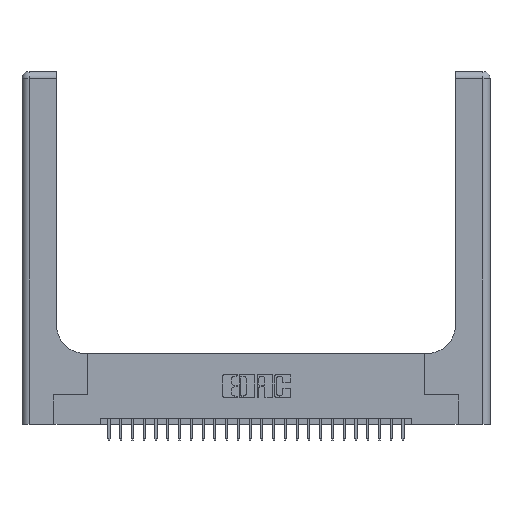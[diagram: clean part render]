
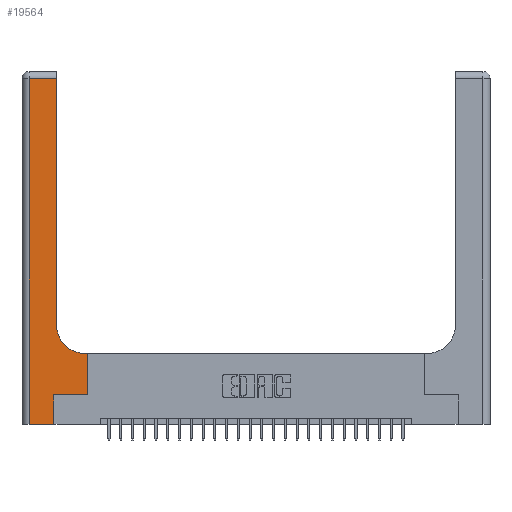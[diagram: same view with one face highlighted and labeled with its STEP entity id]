
A CAD part, top view. The second image highlights one B-rep face of the part: STEP entity #19564.
In plain terms, the highlighted planar face has unit normal (0, 0, 1).
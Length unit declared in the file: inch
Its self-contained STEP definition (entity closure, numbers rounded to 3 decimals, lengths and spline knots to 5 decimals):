
#420 = LINE ( 'NONE', #9033, #13982 ) ;
#2180 = LINE ( 'NONE', #6557, #15878 ) ;
#2312 = DIRECTION ( 'NONE',  ( -1., 0., 0. ) ) ;
#2355 = EDGE_CURVE ( 'NONE', #3383, #12355, #4065, .T. ) ;
#3005 = CARTESIAN_POINT ( 'NONE',  ( 0.5585, 0.6, 0.37 ) ) ;
#3383 = VERTEX_POINT ( 'NONE', #3005 ) ;
#4065 = LINE ( 'NONE', #10394, #23640 ) ;
#4343 = CARTESIAN_POINT ( 'NONE',  ( 0.269, 0., 0.37 ) ) ;
#4801 = CIRCLE ( 'NONE', #18750, 0.25 ) ;
#4947 = DIRECTION ( 'NONE',  ( 0., -1., 0. ) ) ;
#5912 = ORIENTED_EDGE ( 'NONE', *, *, #10742, .T. ) ;
#6061 = DIRECTION ( 'NONE',  ( 1., 0., 0. ) ) ;
#6250 = ORIENTED_EDGE ( 'NONE', *, *, #11276, .T. ) ;
#6557 = CARTESIAN_POINT ( 'NONE',  ( 0.269, 0., 0.37 ) ) ;
#6589 = CARTESIAN_POINT ( 'NONE',  ( 0.2915, 3., 0.37 ) ) ;
#6595 = EDGE_CURVE ( 'NONE', #12355, #13264, #4801, .T. ) ;
#6789 = LINE ( 'NONE', #21723, #9915 ) ;
#7069 = CARTESIAN_POINT ( 'NONE',  ( 0.5415, 0.85, 0.37 ) ) ;
#7431 = CARTESIAN_POINT ( 'NONE',  ( 0.5585, 0.25, 0.37 ) ) ;
#7703 = VECTOR ( 'NONE', #19252, 39.37008 ) ;
#8485 = CARTESIAN_POINT ( 'NONE',  ( 0.2915, 0.85, 0.37 ) ) ;
#8656 = DIRECTION ( 'NONE',  ( 0., 0., -1. ) ) ;
#9033 = CARTESIAN_POINT ( 'NONE',  ( 0., 0., 0.37 ) ) ;
#9044 = EDGE_CURVE ( 'NONE', #11188, #22941, #14479, .T. ) ;
#9915 = VECTOR ( 'NONE', #26227, 39.37008 ) ;
#10226 = DIRECTION ( 'NONE',  ( 1., 0., 0. ) ) ;
#10310 = ORIENTED_EDGE ( 'NONE', *, *, #14823, .T. ) ;
#10365 = CARTESIAN_POINT ( 'NONE',  ( 0., 3., 0.37 ) ) ;
#10394 = CARTESIAN_POINT ( 'NONE',  ( 0.2915, 0.6, 0.37 ) ) ;
#10742 = EDGE_CURVE ( 'NONE', #13264, #24520, #14878, .T. ) ;
#11186 = CARTESIAN_POINT ( 'NONE',  ( 0.2915, 2.94, 0.37 ) ) ;
#11188 = VERTEX_POINT ( 'NONE', #18520 ) ;
#11276 = EDGE_CURVE ( 'NONE', #20802, #11188, #2180, .T. ) ;
#11529 = EDGE_LOOP ( 'NONE', ( #5912, #10310, #25413, #22060, #6250, #22287, #21611, #18761, #16206 ) ) ;
#11717 = EDGE_CURVE ( 'NONE', #25289, #20802, #420, .T. ) ;
#12355 = VERTEX_POINT ( 'NONE', #26466 ) ;
#12738 = VECTOR ( 'NONE', #26748, 39.37008 ) ;
#13264 = VERTEX_POINT ( 'NONE', #8485 ) ;
#13982 = VECTOR ( 'NONE', #10226, 39.37008 ) ;
#14479 = LINE ( 'NONE', #20710, #26351 ) ;
#14733 = EDGE_CURVE ( 'NONE', #19718, #25289, #17744, .T. ) ;
#14823 = EDGE_CURVE ( 'NONE', #24520, #19718, #6789, .T. ) ;
#14878 = LINE ( 'NONE', #6589, #7703 ) ;
#15251 = DIRECTION ( 'NONE',  ( 0., 1., 0. ) ) ;
#15878 = VECTOR ( 'NONE', #15251, 39.37008 ) ;
#16206 = ORIENTED_EDGE ( 'NONE', *, *, #6595, .T. ) ;
#17053 = CARTESIAN_POINT ( 'NONE',  ( 0.06, 0., 0.37 ) ) ;
#17500 = VECTOR ( 'NONE', #4947, 39.37008 ) ;
#17744 = LINE ( 'NONE', #24397, #17500 ) ;
#18520 = CARTESIAN_POINT ( 'NONE',  ( 0.269, 0.25, 0.37 ) ) ;
#18619 = CARTESIAN_POINT ( 'NONE',  ( 0.06, 2.94, 0.37 ) ) ;
#18750 = AXIS2_PLACEMENT_3D ( 'NONE', #7069, #24282, #24694 ) ;
#18761 = ORIENTED_EDGE ( 'NONE', *, *, #2355, .T. ) ;
#18976 = DIRECTION ( 'NONE',  ( -1., 0., 0. ) ) ;
#19252 = DIRECTION ( 'NONE',  ( 0., 1., 0. ) ) ;
#19564 = ADVANCED_FACE ( 'NONE', ( #23201 ), #23476, .F. ) ;
#19718 = VERTEX_POINT ( 'NONE', #18619 ) ;
#20395 = LINE ( 'NONE', #7431, #12738 ) ;
#20710 = CARTESIAN_POINT ( 'NONE',  ( 0.269, 0.25, 0.37 ) ) ;
#20795 = AXIS2_PLACEMENT_3D ( 'NONE', #10365, #8656, #2312 ) ;
#20802 = VERTEX_POINT ( 'NONE', #4343 ) ;
#21611 = ORIENTED_EDGE ( 'NONE', *, *, #23027, .T. ) ;
#21723 = CARTESIAN_POINT ( 'NONE',  ( 0., 2.94, 0.37 ) ) ;
#22060 = ORIENTED_EDGE ( 'NONE', *, *, #11717, .T. ) ;
#22287 = ORIENTED_EDGE ( 'NONE', *, *, #9044, .T. ) ;
#22941 = VERTEX_POINT ( 'NONE', #24372 ) ;
#23027 = EDGE_CURVE ( 'NONE', #22941, #3383, #20395, .T. ) ;
#23201 = FACE_OUTER_BOUND ( 'NONE', #11529, .T. ) ;
#23476 = PLANE ( 'NONE',  #20795 ) ;
#23640 = VECTOR ( 'NONE', #18976, 39.37008 ) ;
#24282 = DIRECTION ( 'NONE',  ( 0., 0., -1. ) ) ;
#24372 = CARTESIAN_POINT ( 'NONE',  ( 0.5585, 0.25, 0.37 ) ) ;
#24397 = CARTESIAN_POINT ( 'NONE',  ( 0.06, 3., 0.37 ) ) ;
#24520 = VERTEX_POINT ( 'NONE', #11186 ) ;
#24694 = DIRECTION ( 'NONE',  ( 1., 0., 0. ) ) ;
#25289 = VERTEX_POINT ( 'NONE', #17053 ) ;
#25413 = ORIENTED_EDGE ( 'NONE', *, *, #14733, .T. ) ;
#26227 = DIRECTION ( 'NONE',  ( -1., 0., 0. ) ) ;
#26351 = VECTOR ( 'NONE', #6061, 39.37008 ) ;
#26466 = CARTESIAN_POINT ( 'NONE',  ( 0.5415, 0.6, 0.37 ) ) ;
#26748 = DIRECTION ( 'NONE',  ( 0., 1., 0. ) ) ;
